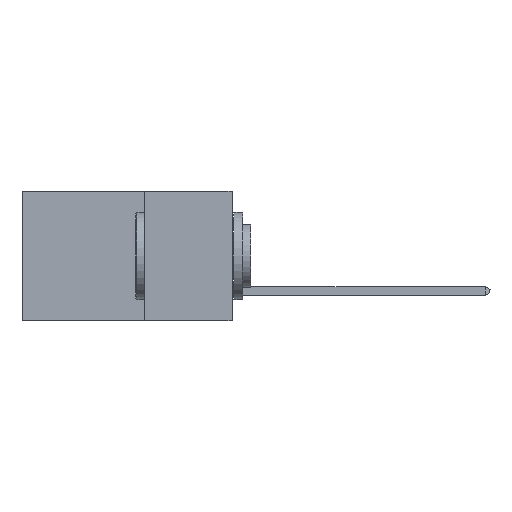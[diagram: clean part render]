
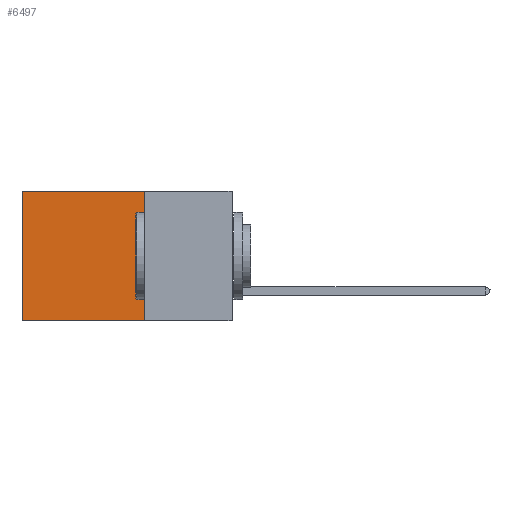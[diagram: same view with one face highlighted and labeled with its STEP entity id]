
A CAD part, left-side view. The second image highlights one B-rep face of the part: STEP entity #6497.
In plain terms, the highlighted planar face has unit normal (-1, 0, 0).
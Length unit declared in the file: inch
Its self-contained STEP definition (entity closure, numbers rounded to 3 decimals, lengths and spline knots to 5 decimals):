
#81 = FACE_OUTER_BOUND ( 'NONE', #24490, .T. ) ;
#733 = ORIENTED_EDGE ( 'NONE', *, *, #17345, .T. ) ;
#3604 = VERTEX_POINT ( 'NONE', #25556 ) ;
#3994 = CARTESIAN_POINT ( 'NONE',  ( 0.2875, 0.25, 0. ) ) ;
#4985 = CARTESIAN_POINT ( 'NONE',  ( 0.2875, 0.6, 0. ) ) ;
#5689 = VECTOR ( 'NONE', #25077, 39.37008 ) ;
#5790 = DIRECTION ( 'NONE',  ( 0., 0., -1. ) ) ;
#6497 = ADVANCED_FACE ( 'NONE', ( #81 ), #21062, .F. ) ;
#7523 = EDGE_CURVE ( 'NONE', #17543, #18634, #22823, .T. ) ;
#7608 = ORIENTED_EDGE ( 'NONE', *, *, #8669, .F. ) ;
#8031 = VECTOR ( 'NONE', #5790, 39.37008 ) ;
#8325 = LINE ( 'NONE', #12128, #5689 ) ;
#8669 = EDGE_CURVE ( 'NONE', #18634, #3604, #8325, .T. ) ;
#10837 = LINE ( 'NONE', #4985, #17236 ) ;
#11940 = EDGE_CURVE ( 'NONE', #17533, #3604, #10837, .T. ) ;
#12109 = DIRECTION ( 'NONE',  ( 0., 0., -1. ) ) ;
#12128 = CARTESIAN_POINT ( 'NONE',  ( 0.2875, 0.25, -0.37 ) ) ;
#13085 = VECTOR ( 'NONE', #22875, 39.37008 ) ;
#13508 = CARTESIAN_POINT ( 'NONE',  ( 0.2875, 0.6, 0. ) ) ;
#13685 = ORIENTED_EDGE ( 'NONE', *, *, #11940, .T. ) ;
#14084 = LINE ( 'NONE', #14323, #13085 ) ;
#14323 = CARTESIAN_POINT ( 'NONE',  ( 0.2875, 0.25, 0. ) ) ;
#15774 = CARTESIAN_POINT ( 'NONE',  ( 0.2875, 0.25, 0. ) ) ;
#16319 = CARTESIAN_POINT ( 'NONE',  ( 0.2875, 0.25, -0.37 ) ) ;
#17236 = VECTOR ( 'NONE', #12109, 39.37008 ) ;
#17345 = EDGE_CURVE ( 'NONE', #17543, #17533, #14084, .T. ) ;
#17533 = VERTEX_POINT ( 'NONE', #13508 ) ;
#17543 = VERTEX_POINT ( 'NONE', #15774 ) ;
#18634 = VERTEX_POINT ( 'NONE', #16319 ) ;
#19090 = DIRECTION ( 'NONE',  ( 1., 0., 0. ) ) ;
#21062 = PLANE ( 'NONE',  #23955 ) ;
#22823 = LINE ( 'NONE', #26970, #8031 ) ;
#22875 = DIRECTION ( 'NONE',  ( 0., 1., 0. ) ) ;
#23312 = DIRECTION ( 'NONE',  ( 0., 0., -1. ) ) ;
#23955 = AXIS2_PLACEMENT_3D ( 'NONE', #3994, #19090, #23312 ) ;
#24226 = ORIENTED_EDGE ( 'NONE', *, *, #7523, .F. ) ;
#24490 = EDGE_LOOP ( 'NONE', ( #13685, #7608, #24226, #733 ) ) ;
#25077 = DIRECTION ( 'NONE',  ( 0., 1., 0. ) ) ;
#25556 = CARTESIAN_POINT ( 'NONE',  ( 0.2875, 0.6, -0.37 ) ) ;
#26970 = CARTESIAN_POINT ( 'NONE',  ( 0.2875, 0.25, 0. ) ) ;
